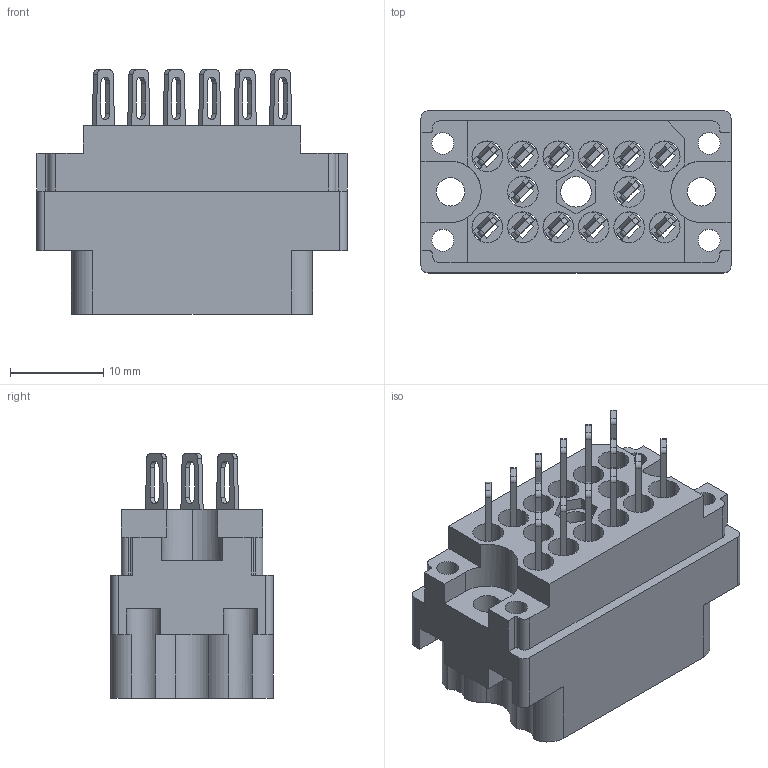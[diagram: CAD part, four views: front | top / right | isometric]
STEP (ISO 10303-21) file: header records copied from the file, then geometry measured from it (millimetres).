
FILE_DESCRIPTION (( 'STEP AP203' ), '1' );
FILE_NAME ('519-014-500-300.STEP', '2020-03-02T19:56:16', ( '' ), ( '' ), 'SwSTEP 2.0', 'SolidWorks 2016', '' );
FILE_SCHEMA (( 'CONFIG_CONTROL_DESIGN' ));
Length unit declared in the file: inch
Products named in the file (3): 516-292-001_500 Contact; 519-014-500-300; 519 Plug Insulator_014
Assembly tree (15 placements, depth 2):
  519-014-500-300
    519 Plug Insulator_014
    516-292-001_500 Contact  x14
Bounding box: 33.32 x 17.42 x 26.26 mm (x, y, z)
Volume: 5478.4 mm3; surface area: 8658.1 mm2
Topology: 15 solids, 15 shells, 1558 faces, 4522 edges, 3004 vertices
Faces by surface type: plane 931, cylinder 541, bspline 84, cone 2
Entity records: 19888 total; most frequent: CARTESIAN_POINT 3641, ORIENTED_EDGE 3324, DIRECTION 3232, EDGE_CURVE 1662, LINE 1188, VECTOR 1188, VERTEX_POINT 1106, AXIS2_PLACEMENT_3D 1022
